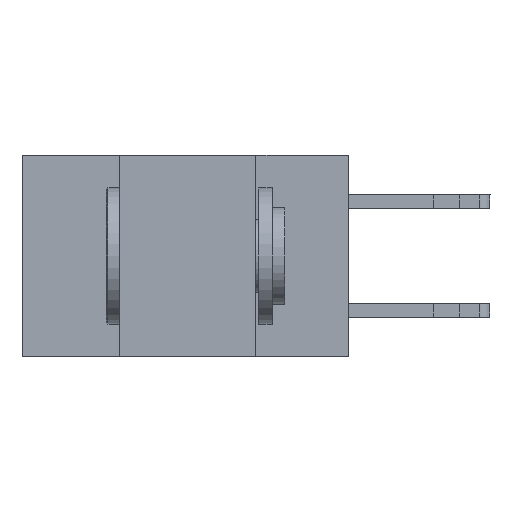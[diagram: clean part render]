
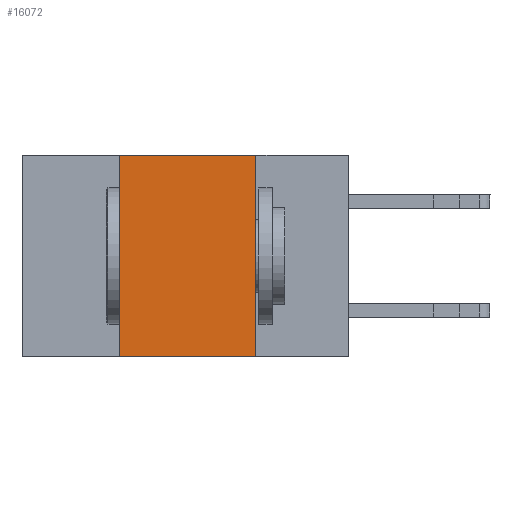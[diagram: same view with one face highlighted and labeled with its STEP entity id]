
A CAD part, left-side view. The second image highlights one B-rep face of the part: STEP entity #16072.
In plain terms, the highlighted planar face has unit normal (-1, 0, 0).
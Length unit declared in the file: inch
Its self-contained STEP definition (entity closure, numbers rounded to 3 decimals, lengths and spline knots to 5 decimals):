
#101 = ORIENTED_EDGE ( 'NONE', *, *, #14401, .F. ) ;
#315 = ORIENTED_EDGE ( 'NONE', *, *, #19118, .T. ) ;
#1166 = VERTEX_POINT ( 'NONE', #16808 ) ;
#1432 = DIRECTION ( 'NONE',  ( 0., -1., 0. ) ) ;
#2252 = ORIENTED_EDGE ( 'NONE', *, *, #21877, .F. ) ;
#2529 = VERTEX_POINT ( 'NONE', #19193 ) ;
#2819 = LINE ( 'NONE', #4662, #22062 ) ;
#3143 = VECTOR ( 'NONE', #15246, 39.37008 ) ;
#3185 = LINE ( 'NONE', #6769, #22906 ) ;
#3280 = LINE ( 'NONE', #8262, #3143 ) ;
#3459 = AXIS2_PLACEMENT_3D ( 'NONE', #5336, #12445, #3608 ) ;
#3608 = DIRECTION ( 'NONE',  ( 0., 0., -1. ) ) ;
#4662 = CARTESIAN_POINT ( 'NONE',  ( 0., 0.6, -0.37 ) ) ;
#5336 = CARTESIAN_POINT ( 'NONE',  ( 0., 0.6, 0. ) ) ;
#6082 = VERTEX_POINT ( 'NONE', #17199 ) ;
#6769 = CARTESIAN_POINT ( 'NONE',  ( 0., 0.6, 0. ) ) ;
#7110 = EDGE_LOOP ( 'NONE', ( #16624, #2252, #101, #315 ) ) ;
#8262 = CARTESIAN_POINT ( 'NONE',  ( 0., 0.17, 0. ) ) ;
#11726 = VERTEX_POINT ( 'NONE', #14869 ) ;
#11775 = DIRECTION ( 'NONE',  ( 0., -1., 0. ) ) ;
#12086 = CARTESIAN_POINT ( 'NONE',  ( 0., 0.42, 0. ) ) ;
#12445 = DIRECTION ( 'NONE',  ( 1., 0., 0. ) ) ;
#13429 = VECTOR ( 'NONE', #22661, 39.37008 ) ;
#14189 = FACE_OUTER_BOUND ( 'NONE', #7110, .T. ) ;
#14401 = EDGE_CURVE ( 'NONE', #6082, #1166, #17298, .T. ) ;
#14869 = CARTESIAN_POINT ( 'NONE',  ( 0., 0.17, 0. ) ) ;
#15246 = DIRECTION ( 'NONE',  ( 0., 0., -1. ) ) ;
#16072 = ADVANCED_FACE ( 'NONE', ( #14189 ), #21272, .F. ) ;
#16624 = ORIENTED_EDGE ( 'NONE', *, *, #19058, .F. ) ;
#16808 = CARTESIAN_POINT ( 'NONE',  ( 0., 0.42, 0. ) ) ;
#17199 = CARTESIAN_POINT ( 'NONE',  ( 0., 0.42, -0.37 ) ) ;
#17298 = LINE ( 'NONE', #12086, #13429 ) ;
#19058 = EDGE_CURVE ( 'NONE', #11726, #2529, #3280, .T. ) ;
#19118 = EDGE_CURVE ( 'NONE', #6082, #2529, #2819, .T. ) ;
#19193 = CARTESIAN_POINT ( 'NONE',  ( 0., 0.17, -0.37 ) ) ;
#21272 = PLANE ( 'NONE',  #3459 ) ;
#21877 = EDGE_CURVE ( 'NONE', #1166, #11726, #3185, .T. ) ;
#22062 = VECTOR ( 'NONE', #11775, 39.37008 ) ;
#22661 = DIRECTION ( 'NONE',  ( 0., 0., 1. ) ) ;
#22906 = VECTOR ( 'NONE', #1432, 39.37008 ) ;
